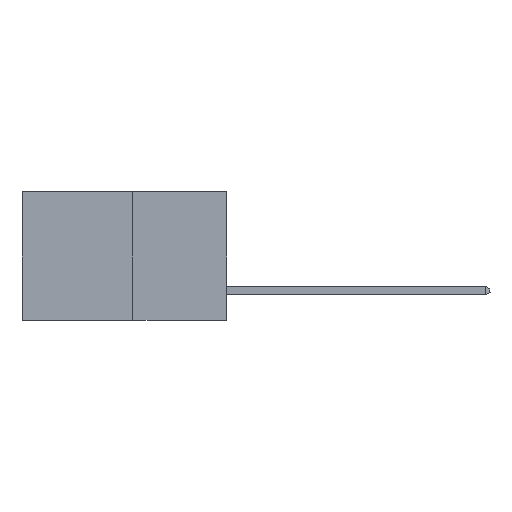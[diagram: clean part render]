
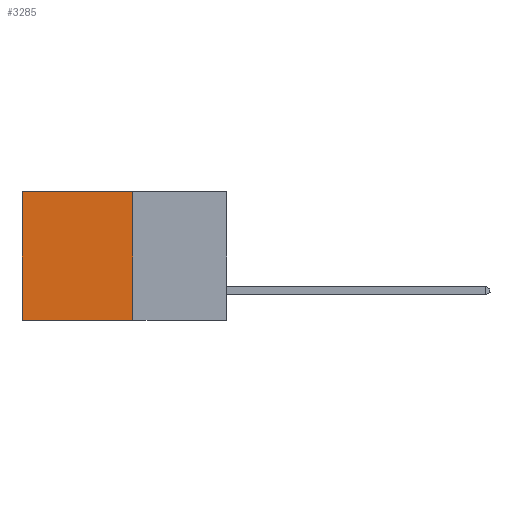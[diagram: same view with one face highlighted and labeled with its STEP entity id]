
A CAD part, left-side view. The second image highlights one B-rep face of the part: STEP entity #3285.
In plain terms, the highlighted planar face has unit normal (-1, 0, 0).
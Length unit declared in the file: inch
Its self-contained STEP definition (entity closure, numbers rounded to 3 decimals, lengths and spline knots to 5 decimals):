
#428 = DIRECTION ( 'NONE',  ( 1., 0., 0. ) ) ;
#874 = AXIS2_PLACEMENT_3D ( 'NONE', #18938, #428, #11203 ) ;
#999 = EDGE_CURVE ( 'NONE', #13628, #13124, #11796, .T. ) ;
#1108 = ORIENTED_EDGE ( 'NONE', *, *, #1304, .F. ) ;
#1304 = EDGE_CURVE ( 'NONE', #11940, #13628, #6466, .T. ) ;
#1514 = CARTESIAN_POINT ( 'NONE',  ( 0.277, 0.27, -0.37 ) ) ;
#1913 = VECTOR ( 'NONE', #5697, 39.37008 ) ;
#1970 = DIRECTION ( 'NONE',  ( 0., 1., 0. ) ) ;
#2836 = EDGE_CURVE ( 'NONE', #11940, #7965, #16359, .T. ) ;
#2962 = VECTOR ( 'NONE', #19549, 39.37008 ) ;
#3285 = ADVANCED_FACE ( 'NONE', ( #15869 ), #8113, .F. ) ;
#3838 = CARTESIAN_POINT ( 'NONE',  ( 0.277, 0.27, -0.37 ) ) ;
#4067 = VECTOR ( 'NONE', #6017, 39.37008 ) ;
#4705 = CARTESIAN_POINT ( 'NONE',  ( 0.277, 0.59, 0. ) ) ;
#5697 = DIRECTION ( 'NONE',  ( 0., 0., -1. ) ) ;
#6017 = DIRECTION ( 'NONE',  ( 0., 1., 0. ) ) ;
#6466 = LINE ( 'NONE', #1514, #1913 ) ;
#6908 = CARTESIAN_POINT ( 'NONE',  ( 0.277, 0.59, -0.37 ) ) ;
#7965 = VERTEX_POINT ( 'NONE', #4705 ) ;
#8113 = PLANE ( 'NONE',  #874 ) ;
#8115 = VECTOR ( 'NONE', #1970, 39.37008 ) ;
#9156 = EDGE_CURVE ( 'NONE', #7965, #13124, #11153, .T. ) ;
#9403 = ORIENTED_EDGE ( 'NONE', *, *, #9156, .T. ) ;
#9467 = CARTESIAN_POINT ( 'NONE',  ( 0.277, 0.27, 0. ) ) ;
#11153 = LINE ( 'NONE', #6908, #2962 ) ;
#11203 = DIRECTION ( 'NONE',  ( 0., 0., -1. ) ) ;
#11467 = CARTESIAN_POINT ( 'NONE',  ( 0.277, 0.27, -0.37 ) ) ;
#11796 = LINE ( 'NONE', #3838, #4067 ) ;
#11833 = CARTESIAN_POINT ( 'NONE',  ( 0.277, 0.59, -0.37 ) ) ;
#11940 = VERTEX_POINT ( 'NONE', #15376 ) ;
#13025 = EDGE_LOOP ( 'NONE', ( #9403, #17648, #1108, #14246 ) ) ;
#13124 = VERTEX_POINT ( 'NONE', #11833 ) ;
#13628 = VERTEX_POINT ( 'NONE', #11467 ) ;
#14246 = ORIENTED_EDGE ( 'NONE', *, *, #2836, .T. ) ;
#15376 = CARTESIAN_POINT ( 'NONE',  ( 0.277, 0.27, 0. ) ) ;
#15869 = FACE_OUTER_BOUND ( 'NONE', #13025, .T. ) ;
#16359 = LINE ( 'NONE', #9467, #8115 ) ;
#17648 = ORIENTED_EDGE ( 'NONE', *, *, #999, .F. ) ;
#18938 = CARTESIAN_POINT ( 'NONE',  ( 0.277, 0.27, -0.37 ) ) ;
#19549 = DIRECTION ( 'NONE',  ( 0., 0., -1. ) ) ;
